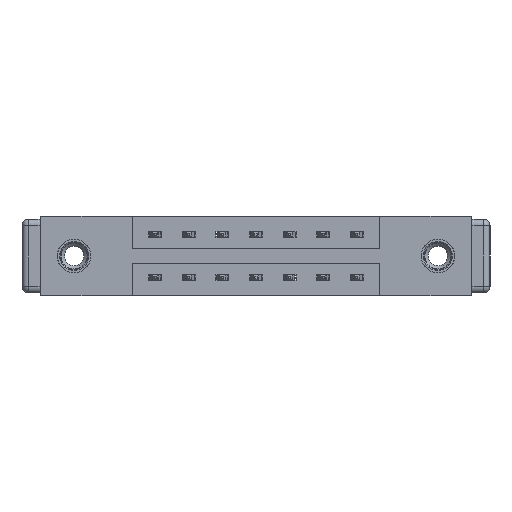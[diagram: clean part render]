
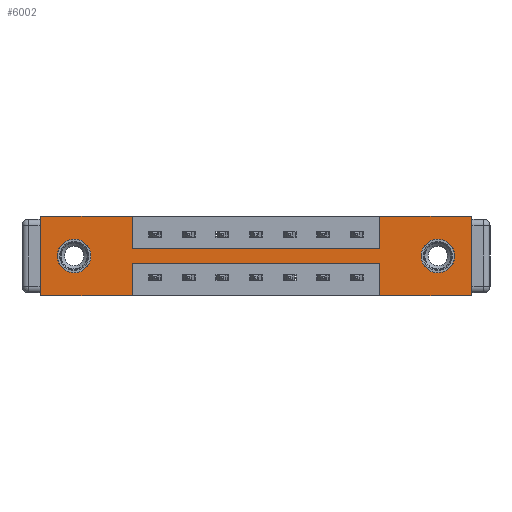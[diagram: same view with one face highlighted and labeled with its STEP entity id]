
A CAD part, front view. The second image highlights one B-rep face of the part: STEP entity #6002.
In plain terms, the highlighted planar face has unit normal (0, -1, 0).
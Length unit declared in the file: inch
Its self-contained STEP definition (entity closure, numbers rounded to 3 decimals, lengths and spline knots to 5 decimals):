
#3 = ORIENTED_EDGE ( 'NONE', *, *, #10673, .T. ) ;
#89 = CARTESIAN_POINT ( 'NONE',  ( 0.425, 0., -0.22 ) ) ;
#207 = EDGE_LOOP ( 'NONE', ( #5360, #847 ) ) ;
#209 = PLANE ( 'NONE',  #5074 ) ;
#218 = EDGE_LOOP ( 'NONE', ( #1865, #10202, #8437, #1012, #4181, #2950, #3966, #8333, #2251, #6210, #5039, #2558 ) ) ;
#245 = DIRECTION ( 'NONE',  ( 0., -1., 0. ) ) ;
#513 = CARTESIAN_POINT ( 'NONE',  ( 1.573, 0., 0. ) ) ;
#847 = ORIENTED_EDGE ( 'NONE', *, *, #4902, .T. ) ;
#995 = CARTESIAN_POINT ( 'NONE',  ( 1.573, 0., -0.15 ) ) ;
#1005 = CARTESIAN_POINT ( 'NONE',  ( 0., 0., -0.37 ) ) ;
#1012 = ORIENTED_EDGE ( 'NONE', *, *, #12362, .F. ) ;
#1133 = VERTEX_POINT ( 'NONE', #3407 ) ;
#1154 = LINE ( 'NONE', #10969, #3756 ) ;
#1176 = CARTESIAN_POINT ( 'NONE',  ( 0.425, 0., -0.37 ) ) ;
#1287 = EDGE_CURVE ( 'NONE', #1133, #10456, #10665, .T. ) ;
#1399 = LINE ( 'NONE', #89, #8484 ) ;
#1589 = VERTEX_POINT ( 'NONE', #995 ) ;
#1692 = CARTESIAN_POINT ( 'NONE',  ( 1.843, 0., -0.185 ) ) ;
#1799 = LINE ( 'NONE', #9153, #6232 ) ;
#1821 = DIRECTION ( 'NONE',  ( -1., 0., 0. ) ) ;
#1823 = AXIS2_PLACEMENT_3D ( 'NONE', #7856, #8456, #2575 ) ;
#1859 = FACE_BOUND ( 'NONE', #207, .T. ) ;
#1865 = ORIENTED_EDGE ( 'NONE', *, *, #1287, .F. ) ;
#2079 = VERTEX_POINT ( 'NONE', #5618 ) ;
#2117 = VERTEX_POINT ( 'NONE', #5474 ) ;
#2158 = FACE_BOUND ( 'NONE', #6321, .T. ) ;
#2251 = ORIENTED_EDGE ( 'NONE', *, *, #3734, .F. ) ;
#2558 = ORIENTED_EDGE ( 'NONE', *, *, #4696, .F. ) ;
#2568 = CARTESIAN_POINT ( 'NONE',  ( 1.998, 0., -0.37 ) ) ;
#2575 = DIRECTION ( 'NONE',  ( 0., 0., -1. ) ) ;
#2648 = DIRECTION ( 'NONE',  ( 1., 0., 0. ) ) ;
#2786 = VECTOR ( 'NONE', #6008, 39.37008 ) ;
#2787 = CARTESIAN_POINT ( 'NONE',  ( 0., 0., -0.37 ) ) ;
#2808 = EDGE_CURVE ( 'NONE', #4674, #9033, #10181, .T. ) ;
#2941 = AXIS2_PLACEMENT_3D ( 'NONE', #4257, #12115, #5525 ) ;
#2948 = VECTOR ( 'NONE', #5031, 39.37008 ) ;
#2950 = ORIENTED_EDGE ( 'NONE', *, *, #11608, .F. ) ;
#3081 = FACE_OUTER_BOUND ( 'NONE', #218, .T. ) ;
#3147 = CARTESIAN_POINT ( 'NONE',  ( 1.998, 0., 0. ) ) ;
#3302 = LINE ( 'NONE', #9138, #10842 ) ;
#3407 = CARTESIAN_POINT ( 'NONE',  ( 0.425, 0., -0.22 ) ) ;
#3531 = EDGE_CURVE ( 'NONE', #11908, #12051, #9233, .T. ) ;
#3734 = EDGE_CURVE ( 'NONE', #7484, #8276, #8150, .T. ) ;
#3756 = VECTOR ( 'NONE', #9101, 39.37008 ) ;
#3966 = ORIENTED_EDGE ( 'NONE', *, *, #10280, .F. ) ;
#3984 = VECTOR ( 'NONE', #12380, 39.37008 ) ;
#4011 = LINE ( 'NONE', #5535, #5476 ) ;
#4012 = VERTEX_POINT ( 'NONE', #2787 ) ;
#4035 = VERTEX_POINT ( 'NONE', #7766 ) ;
#4154 = CARTESIAN_POINT ( 'NONE',  ( 1.573, 0., -0.37 ) ) ;
#4181 = ORIENTED_EDGE ( 'NONE', *, *, #3531, .F. ) ;
#4257 = CARTESIAN_POINT ( 'NONE',  ( 0.155, 0., -0.185 ) ) ;
#4276 = VECTOR ( 'NONE', #2648, 39.37008 ) ;
#4393 = VERTEX_POINT ( 'NONE', #4154 ) ;
#4674 = VERTEX_POINT ( 'NONE', #10848 ) ;
#4696 = EDGE_CURVE ( 'NONE', #10456, #4012, #9196, .T. ) ;
#4902 = EDGE_CURVE ( 'NONE', #9033, #4674, #8428, .T. ) ;
#5031 = DIRECTION ( 'NONE',  ( 0., 0., -1. ) ) ;
#5039 = ORIENTED_EDGE ( 'NONE', *, *, #9298, .F. ) ;
#5074 = AXIS2_PLACEMENT_3D ( 'NONE', #7093, #245, #10948 ) ;
#5360 = ORIENTED_EDGE ( 'NONE', *, *, #2808, .T. ) ;
#5474 = CARTESIAN_POINT ( 'NONE',  ( 1.843, 0., -0.263 ) ) ;
#5476 = VECTOR ( 'NONE', #10306, 39.37008 ) ;
#5525 = DIRECTION ( 'NONE',  ( 0., 0., 1. ) ) ;
#5535 = CARTESIAN_POINT ( 'NONE',  ( 0., 0., 0. ) ) ;
#5549 = VECTOR ( 'NONE', #1821, 39.37008 ) ;
#5618 = CARTESIAN_POINT ( 'NONE',  ( 1.843, 0., -0.107 ) ) ;
#6002 = ADVANCED_FACE ( 'NONE', ( #2158, #1859, #3081 ), #209, .T. ) ;
#6008 = DIRECTION ( 'NONE',  ( 0., 0., -1. ) ) ;
#6210 = ORIENTED_EDGE ( 'NONE', *, *, #12235, .F. ) ;
#6232 = VECTOR ( 'NONE', #11203, 39.37008 ) ;
#6321 = EDGE_LOOP ( 'NONE', ( #3, #10366 ) ) ;
#6350 = AXIS2_PLACEMENT_3D ( 'NONE', #9758, #10720, #10771 ) ;
#6761 = DIRECTION ( 'NONE',  ( 0., 0., -1. ) ) ;
#6845 = DIRECTION ( 'NONE',  ( 0., 0., 1. ) ) ;
#7093 = CARTESIAN_POINT ( 'NONE',  ( 0., 0., -0.37 ) ) ;
#7101 = EDGE_CURVE ( 'NONE', #4393, #7549, #1799, .T. ) ;
#7479 = CARTESIAN_POINT ( 'NONE',  ( 1.573, 0., 0. ) ) ;
#7484 = VERTEX_POINT ( 'NONE', #10337 ) ;
#7525 = DIRECTION ( 'NONE',  ( 0., 1., 0. ) ) ;
#7549 = VERTEX_POINT ( 'NONE', #10507 ) ;
#7643 = CIRCLE ( 'NONE', #7994, 0.078 ) ;
#7766 = CARTESIAN_POINT ( 'NONE',  ( 0., 0., 0. ) ) ;
#7856 = CARTESIAN_POINT ( 'NONE',  ( 1.843, 0., -0.185 ) ) ;
#7978 = CARTESIAN_POINT ( 'NONE',  ( 0.425, 0., 0. ) ) ;
#7994 = AXIS2_PLACEMENT_3D ( 'NONE', #1692, #7525, #10573 ) ;
#8150 = LINE ( 'NONE', #7978, #2786 ) ;
#8276 = VERTEX_POINT ( 'NONE', #8545 ) ;
#8333 = ORIENTED_EDGE ( 'NONE', *, *, #10205, .F. ) ;
#8428 = CIRCLE ( 'NONE', #2941, 0.078 ) ;
#8437 = ORIENTED_EDGE ( 'NONE', *, *, #7101, .F. ) ;
#8456 = DIRECTION ( 'NONE',  ( 0., 1., 0. ) ) ;
#8484 = VECTOR ( 'NONE', #10918, 39.37008 ) ;
#8545 = CARTESIAN_POINT ( 'NONE',  ( 0.425, 0., -0.15 ) ) ;
#8659 = CARTESIAN_POINT ( 'NONE',  ( 0.155, 0., -0.263 ) ) ;
#8794 = VERTEX_POINT ( 'NONE', #513 ) ;
#9033 = VERTEX_POINT ( 'NONE', #8659 ) ;
#9101 = DIRECTION ( 'NONE',  ( 1., 0., 0. ) ) ;
#9138 = CARTESIAN_POINT ( 'NONE',  ( 0., 0., 0. ) ) ;
#9153 = CARTESIAN_POINT ( 'NONE',  ( 1.573, 0., -0.37 ) ) ;
#9193 = VECTOR ( 'NONE', #6845, 39.37008 ) ;
#9196 = LINE ( 'NONE', #12567, #3984 ) ;
#9233 = LINE ( 'NONE', #3147, #2948 ) ;
#9298 = EDGE_CURVE ( 'NONE', #4012, #4035, #4011, .T. ) ;
#9655 = LINE ( 'NONE', #12423, #4276 ) ;
#9758 = CARTESIAN_POINT ( 'NONE',  ( 0.155, 0., -0.185 ) ) ;
#9878 = LINE ( 'NONE', #1005, #5549 ) ;
#10171 = EDGE_CURVE ( 'NONE', #2117, #2079, #7643, .T. ) ;
#10181 = CIRCLE ( 'NONE', #6350, 0.078 ) ;
#10202 = ORIENTED_EDGE ( 'NONE', *, *, #12508, .F. ) ;
#10205 = EDGE_CURVE ( 'NONE', #8276, #1589, #9655, .T. ) ;
#10280 = EDGE_CURVE ( 'NONE', #1589, #8794, #12254, .T. ) ;
#10306 = DIRECTION ( 'NONE',  ( 0., 0., 1. ) ) ;
#10337 = CARTESIAN_POINT ( 'NONE',  ( 0.425, 0., 0. ) ) ;
#10339 = VECTOR ( 'NONE', #6761, 39.37008 ) ;
#10366 = ORIENTED_EDGE ( 'NONE', *, *, #10171, .T. ) ;
#10456 = VERTEX_POINT ( 'NONE', #1176 ) ;
#10507 = CARTESIAN_POINT ( 'NONE',  ( 1.573, 0., -0.22 ) ) ;
#10573 = DIRECTION ( 'NONE',  ( 0., 0., -1. ) ) ;
#10622 = CARTESIAN_POINT ( 'NONE',  ( 0.425, 0., -0.37 ) ) ;
#10665 = LINE ( 'NONE', #10622, #10339 ) ;
#10673 = EDGE_CURVE ( 'NONE', #2079, #2117, #12400, .T. ) ;
#10720 = DIRECTION ( 'NONE',  ( 0., 1., 0. ) ) ;
#10771 = DIRECTION ( 'NONE',  ( 0., 0., 1. ) ) ;
#10842 = VECTOR ( 'NONE', #12026, 39.37008 ) ;
#10848 = CARTESIAN_POINT ( 'NONE',  ( 0.155, 0., -0.107 ) ) ;
#10918 = DIRECTION ( 'NONE',  ( -1., 0., 0. ) ) ;
#10948 = DIRECTION ( 'NONE',  ( 0., 0., -1. ) ) ;
#10969 = CARTESIAN_POINT ( 'NONE',  ( 0., 0., 0. ) ) ;
#11203 = DIRECTION ( 'NONE',  ( 0., 0., 1. ) ) ;
#11608 = EDGE_CURVE ( 'NONE', #8794, #11908, #3302, .T. ) ;
#11715 = CARTESIAN_POINT ( 'NONE',  ( 1.998, 0., 0. ) ) ;
#11908 = VERTEX_POINT ( 'NONE', #11715 ) ;
#12026 = DIRECTION ( 'NONE',  ( 1., 0., 0. ) ) ;
#12051 = VERTEX_POINT ( 'NONE', #2568 ) ;
#12115 = DIRECTION ( 'NONE',  ( 0., 1., 0. ) ) ;
#12235 = EDGE_CURVE ( 'NONE', #4035, #7484, #1154, .T. ) ;
#12254 = LINE ( 'NONE', #7479, #9193 ) ;
#12362 = EDGE_CURVE ( 'NONE', #12051, #4393, #9878, .T. ) ;
#12380 = DIRECTION ( 'NONE',  ( -1., 0., 0. ) ) ;
#12400 = CIRCLE ( 'NONE', #1823, 0.078 ) ;
#12423 = CARTESIAN_POINT ( 'NONE',  ( 0.425, 0., -0.15 ) ) ;
#12508 = EDGE_CURVE ( 'NONE', #7549, #1133, #1399, .T. ) ;
#12567 = CARTESIAN_POINT ( 'NONE',  ( 0., 0., -0.37 ) ) ;
